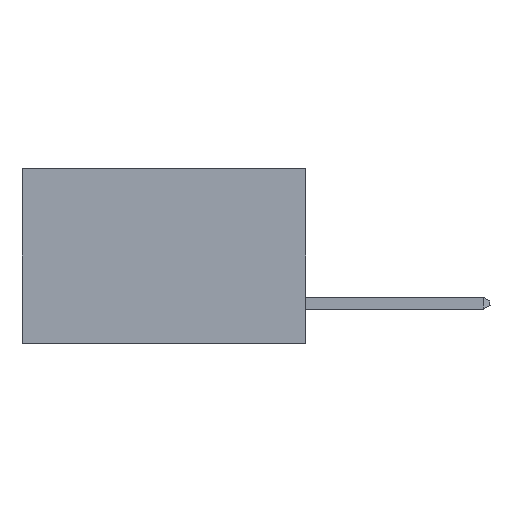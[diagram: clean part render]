
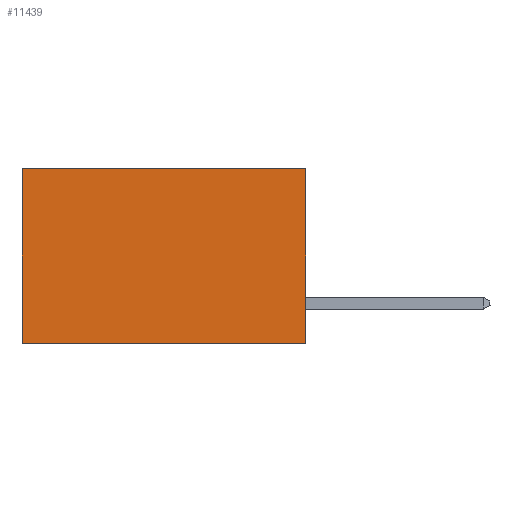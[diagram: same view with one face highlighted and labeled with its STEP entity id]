
A CAD part, left-side view. The second image highlights one B-rep face of the part: STEP entity #11439.
In plain terms, the highlighted planar face has unit normal (-1, 0, 0).
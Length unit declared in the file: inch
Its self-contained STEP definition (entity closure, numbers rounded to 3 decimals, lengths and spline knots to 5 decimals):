
#405 = EDGE_CURVE ( 'NONE', #10059, #7464, #11801, .T. ) ;
#441 = ORIENTED_EDGE ( 'NONE', *, *, #12147, .F. ) ;
#723 = EDGE_CURVE ( 'NONE', #7275, #12944, #5184, .T. ) ;
#966 = AXIS2_PLACEMENT_3D ( 'NONE', #10004, #3376, #11163 ) ;
#1070 = LINE ( 'NONE', #1193, #3294 ) ;
#1193 = CARTESIAN_POINT ( 'NONE',  ( 0.298, 0., 0. ) ) ;
#1337 = DIRECTION ( 'NONE',  ( 0., 1., 0. ) ) ;
#2244 = PLANE ( 'NONE',  #966 ) ;
#2395 = DIRECTION ( 'NONE',  ( 0., 1., 0. ) ) ;
#2546 = ORIENTED_EDGE ( 'NONE', *, *, #405, .T. ) ;
#3294 = VECTOR ( 'NONE', #2395, 39.37008 ) ;
#3376 = DIRECTION ( 'NONE',  ( 1., 0., 0. ) ) ;
#4547 = CARTESIAN_POINT ( 'NONE',  ( 0.298, 0., -0.37 ) ) ;
#5184 = LINE ( 'NONE', #5644, #6593 ) ;
#5542 = VECTOR ( 'NONE', #7204, 39.37008 ) ;
#5644 = CARTESIAN_POINT ( 'NONE',  ( 0.298, 0., 0. ) ) ;
#5688 = CARTESIAN_POINT ( 'NONE',  ( 0.298, 0.6, -0.37 ) ) ;
#5693 = ORIENTED_EDGE ( 'NONE', *, *, #723, .F. ) ;
#6341 = LINE ( 'NONE', #4547, #12427 ) ;
#6593 = VECTOR ( 'NONE', #9221, 39.37008 ) ;
#6810 = CARTESIAN_POINT ( 'NONE',  ( 0.298, 0., -0.37 ) ) ;
#6976 = CARTESIAN_POINT ( 'NONE',  ( 0.298, 0.6, 0. ) ) ;
#7068 = FACE_OUTER_BOUND ( 'NONE', #9134, .T. ) ;
#7204 = DIRECTION ( 'NONE',  ( 0., 0., -1. ) ) ;
#7275 = VERTEX_POINT ( 'NONE', #12782 ) ;
#7464 = VERTEX_POINT ( 'NONE', #5688 ) ;
#9134 = EDGE_LOOP ( 'NONE', ( #2546, #441, #5693, #13858 ) ) ;
#9195 = CARTESIAN_POINT ( 'NONE',  ( 0.298, 0.6, 0. ) ) ;
#9221 = DIRECTION ( 'NONE',  ( 0., 0., -1. ) ) ;
#9863 = EDGE_CURVE ( 'NONE', #7275, #10059, #1070, .T. ) ;
#10004 = CARTESIAN_POINT ( 'NONE',  ( 0.298, 0., 0. ) ) ;
#10059 = VERTEX_POINT ( 'NONE', #9195 ) ;
#11163 = DIRECTION ( 'NONE',  ( 0., 0., -1. ) ) ;
#11439 = ADVANCED_FACE ( 'NONE', ( #7068 ), #2244, .F. ) ;
#11801 = LINE ( 'NONE', #6976, #5542 ) ;
#12147 = EDGE_CURVE ( 'NONE', #12944, #7464, #6341, .T. ) ;
#12427 = VECTOR ( 'NONE', #1337, 39.37008 ) ;
#12782 = CARTESIAN_POINT ( 'NONE',  ( 0.298, 0., 0. ) ) ;
#12944 = VERTEX_POINT ( 'NONE', #6810 ) ;
#13858 = ORIENTED_EDGE ( 'NONE', *, *, #9863, .T. ) ;
